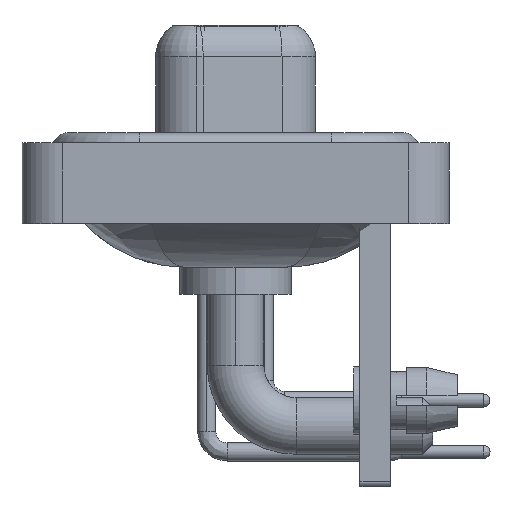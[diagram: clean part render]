
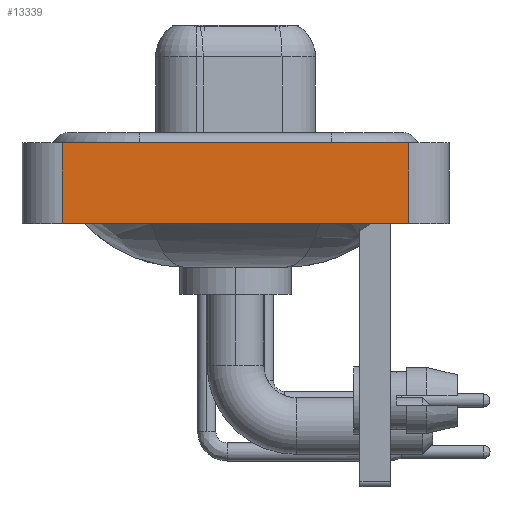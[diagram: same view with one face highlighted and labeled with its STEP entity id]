
A CAD part, left-side view. The second image highlights one B-rep face of the part: STEP entity #13339.
In plain terms, the highlighted planar face has unit normal (-1, 0, 0).
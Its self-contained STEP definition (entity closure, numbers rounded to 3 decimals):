
#199 = LINE ( 'NONE', #2329, #4995 ) ;
#237 = CARTESIAN_POINT ( 'NONE',  ( -7.35, 8.55, -3.6 ) ) ;
#1698 = EDGE_CURVE ( 'NONE', #8464, #22090, #199, .T. ) ;
#1882 = FACE_OUTER_BOUND ( 'NONE', #19813, .T. ) ;
#1992 = CARTESIAN_POINT ( 'NONE',  ( -7.35, 8.55, -3.6 ) ) ;
#2329 = CARTESIAN_POINT ( 'NONE',  ( -7.35, -8.55, -3.6 ) ) ;
#2504 = LINE ( 'NONE', #9706, #21006 ) ;
#3673 = PLANE ( 'NONE',  #4850 ) ;
#4219 = EDGE_CURVE ( 'NONE', #8464, #13060, #12907, .T. ) ;
#4382 = CARTESIAN_POINT ( 'NONE',  ( -7.35, -8.55, -3.6 ) ) ;
#4850 = AXIS2_PLACEMENT_3D ( 'NONE', #12776, #10860, #16498 ) ;
#4995 = VECTOR ( 'NONE', #5411, 1000. ) ;
#5411 = DIRECTION ( 'NONE',  ( 0., -1., 0. ) ) ;
#7185 = EDGE_CURVE ( 'NONE', #22090, #13447, #9386, .T. ) ;
#8464 = VERTEX_POINT ( 'NONE', #1992 ) ;
#9386 = LINE ( 'NONE', #20437, #10336 ) ;
#9706 = CARTESIAN_POINT ( 'NONE',  ( -7.35, -8.55, 0.4 ) ) ;
#9930 = ORIENTED_EDGE ( 'NONE', *, *, #1698, .T. ) ;
#10336 = VECTOR ( 'NONE', #15101, 1000. ) ;
#10860 = DIRECTION ( 'NONE',  ( -1., 0., 0. ) ) ;
#10972 = ORIENTED_EDGE ( 'NONE', *, *, #17367, .F. ) ;
#12776 = CARTESIAN_POINT ( 'NONE',  ( -7.35, -8.55, -3.6 ) ) ;
#12907 = LINE ( 'NONE', #237, #14443 ) ;
#13060 = VERTEX_POINT ( 'NONE', #13417 ) ;
#13339 = ADVANCED_FACE ( 'NONE', ( #1882 ), #3673, .T. ) ;
#13417 = CARTESIAN_POINT ( 'NONE',  ( -7.35, 8.55, 0.4 ) ) ;
#13447 = VERTEX_POINT ( 'NONE', #20737 ) ;
#14443 = VECTOR ( 'NONE', #14696, 1000. ) ;
#14696 = DIRECTION ( 'NONE',  ( 0., 0., 1. ) ) ;
#15101 = DIRECTION ( 'NONE',  ( 0., 0., 1. ) ) ;
#16498 = DIRECTION ( 'NONE',  ( 0., 0., 1. ) ) ;
#17192 = ORIENTED_EDGE ( 'NONE', *, *, #4219, .F. ) ;
#17367 = EDGE_CURVE ( 'NONE', #13060, #13447, #2504, .T. ) ;
#19813 = EDGE_LOOP ( 'NONE', ( #22708, #10972, #17192, #9930 ) ) ;
#20437 = CARTESIAN_POINT ( 'NONE',  ( -7.35, -8.55, -3.6 ) ) ;
#20737 = CARTESIAN_POINT ( 'NONE',  ( -7.35, -8.55, 0.4 ) ) ;
#21006 = VECTOR ( 'NONE', #22428, 1000. ) ;
#22090 = VERTEX_POINT ( 'NONE', #4382 ) ;
#22428 = DIRECTION ( 'NONE',  ( 0., -1., 0. ) ) ;
#22708 = ORIENTED_EDGE ( 'NONE', *, *, #7185, .T. ) ;
